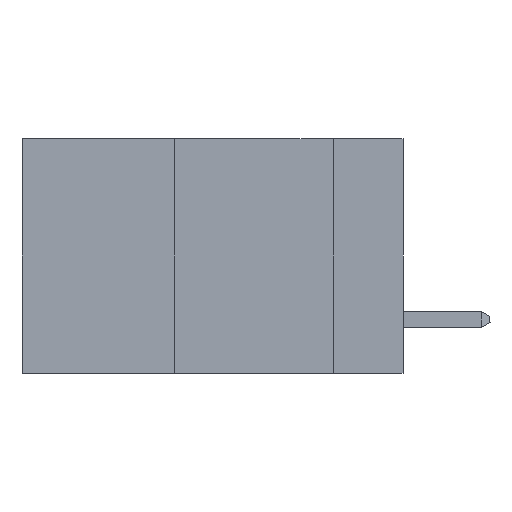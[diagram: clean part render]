
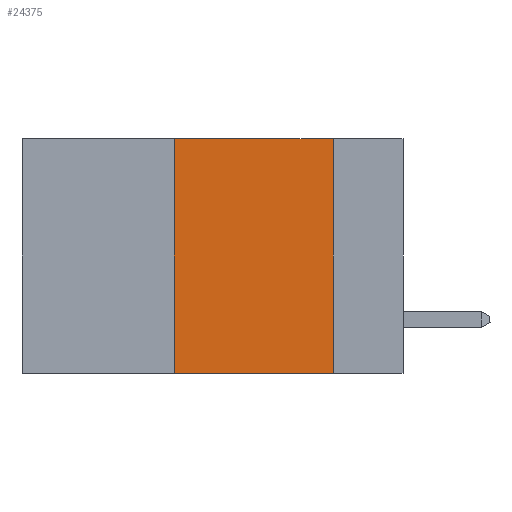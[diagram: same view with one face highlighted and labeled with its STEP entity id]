
A CAD part, left-side view. The second image highlights one B-rep face of the part: STEP entity #24375.
In plain terms, the highlighted planar face has unit normal (-1, 0, 0).
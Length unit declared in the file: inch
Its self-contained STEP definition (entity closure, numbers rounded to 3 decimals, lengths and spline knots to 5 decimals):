
#427 = CARTESIAN_POINT ( 'NONE',  ( 0., 0.36, 0. ) ) ;
#595 = DIRECTION ( 'NONE',  ( 0., 0., -1. ) ) ;
#844 = EDGE_CURVE ( 'NONE', #10476, #4553, #22180, .T. ) ;
#2294 = EDGE_CURVE ( 'NONE', #10988, #4553, #16014, .T. ) ;
#2348 = VECTOR ( 'NONE', #26351, 39.37008 ) ;
#4345 = VECTOR ( 'NONE', #31974, 39.37008 ) ;
#4553 = VERTEX_POINT ( 'NONE', #6053 ) ;
#5087 = CARTESIAN_POINT ( 'NONE',  ( 0., 0.11, 0. ) ) ;
#6053 = CARTESIAN_POINT ( 'NONE',  ( 0., 0.11, -0.37 ) ) ;
#6882 = VECTOR ( 'NONE', #14881, 39.37008 ) ;
#7698 = ORIENTED_EDGE ( 'NONE', *, *, #2294, .F. ) ;
#7772 = ORIENTED_EDGE ( 'NONE', *, *, #13477, .F. ) ;
#8530 = EDGE_LOOP ( 'NONE', ( #7698, #18786, #7772, #9357 ) ) ;
#9357 = ORIENTED_EDGE ( 'NONE', *, *, #844, .T. ) ;
#9803 = CARTESIAN_POINT ( 'NONE',  ( 0., 0.6, -0.37 ) ) ;
#9829 = DIRECTION ( 'NONE',  ( 0., 0., -1. ) ) ;
#10476 = VERTEX_POINT ( 'NONE', #21691 ) ;
#10988 = VERTEX_POINT ( 'NONE', #22165 ) ;
#12470 = FACE_OUTER_BOUND ( 'NONE', #8530, .T. ) ;
#13477 = EDGE_CURVE ( 'NONE', #10476, #20944, #19297, .T. ) ;
#14193 = DIRECTION ( 'NONE',  ( 1., 0., 0. ) ) ;
#14438 = EDGE_CURVE ( 'NONE', #20944, #10988, #27400, .T. ) ;
#14881 = DIRECTION ( 'NONE',  ( 0., -1., 0. ) ) ;
#16014 = LINE ( 'NONE', #5087, #20465 ) ;
#18786 = ORIENTED_EDGE ( 'NONE', *, *, #14438, .F. ) ;
#19297 = LINE ( 'NONE', #427, #4345 ) ;
#20465 = VECTOR ( 'NONE', #9829, 39.37008 ) ;
#20944 = VERTEX_POINT ( 'NONE', #24299 ) ;
#21691 = CARTESIAN_POINT ( 'NONE',  ( 0., 0.36, -0.37 ) ) ;
#22165 = CARTESIAN_POINT ( 'NONE',  ( 0., 0.11, 0. ) ) ;
#22180 = LINE ( 'NONE', #9803, #6882 ) ;
#24299 = CARTESIAN_POINT ( 'NONE',  ( 0., 0.36, 0. ) ) ;
#24375 = ADVANCED_FACE ( 'NONE', ( #12470 ), #26135, .F. ) ;
#24845 = AXIS2_PLACEMENT_3D ( 'NONE', #29007, #14193, #595 ) ;
#26135 = PLANE ( 'NONE',  #24845 ) ;
#26351 = DIRECTION ( 'NONE',  ( 0., -1., 0. ) ) ;
#27400 = LINE ( 'NONE', #28671, #2348 ) ;
#28671 = CARTESIAN_POINT ( 'NONE',  ( 0., 0.6, 0. ) ) ;
#29007 = CARTESIAN_POINT ( 'NONE',  ( 0., 0.6, 0. ) ) ;
#31974 = DIRECTION ( 'NONE',  ( 0., 0., 1. ) ) ;
